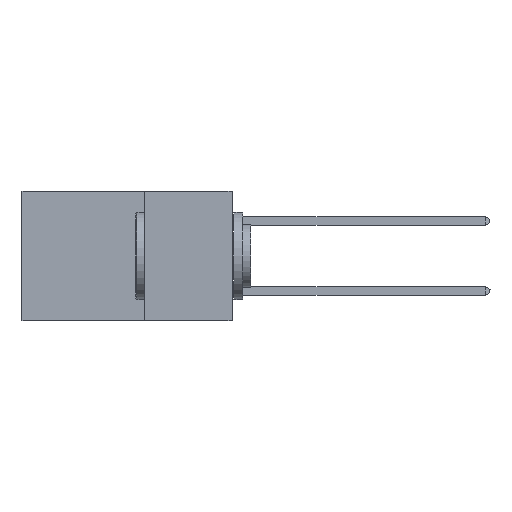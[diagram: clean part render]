
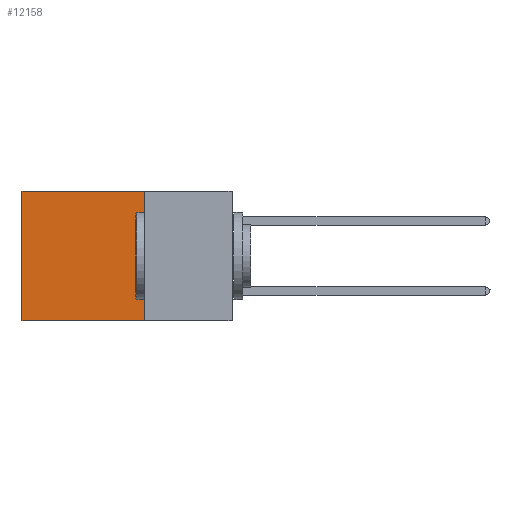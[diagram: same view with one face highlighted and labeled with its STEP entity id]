
A CAD part, left-side view. The second image highlights one B-rep face of the part: STEP entity #12158.
In plain terms, the highlighted planar face has unit normal (-1, 0, 0).
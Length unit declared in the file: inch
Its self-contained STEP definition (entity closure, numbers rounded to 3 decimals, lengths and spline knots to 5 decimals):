
#1408 = CARTESIAN_POINT ( 'NONE',  ( 0.2875, 0.25, 0. ) ) ;
#3060 = VECTOR ( 'NONE', #18854, 39.37008 ) ;
#3437 = ORIENTED_EDGE ( 'NONE', *, *, #14255, .F. ) ;
#5134 = ORIENTED_EDGE ( 'NONE', *, *, #11934, .F. ) ;
#6061 = ORIENTED_EDGE ( 'NONE', *, *, #16814, .T. ) ;
#7436 = FACE_OUTER_BOUND ( 'NONE', #12693, .T. ) ;
#8294 = LINE ( 'NONE', #42386, #42896 ) ;
#11934 = EDGE_CURVE ( 'NONE', #23235, #21359, #41029, .T. ) ;
#12158 = ADVANCED_FACE ( 'NONE', ( #7436 ), #16274, .F. ) ;
#12693 = EDGE_LOOP ( 'NONE', ( #6061, #3437, #5134, #21811 ) ) ;
#12877 = LINE ( 'NONE', #31727, #30169 ) ;
#14255 = EDGE_CURVE ( 'NONE', #21359, #35211, #8294, .T. ) ;
#14597 = LINE ( 'NONE', #27850, #3060 ) ;
#15243 = CARTESIAN_POINT ( 'NONE',  ( 0.2875, 0.6, 0. ) ) ;
#16274 = PLANE ( 'NONE',  #39354 ) ;
#16450 = VECTOR ( 'NONE', #43091, 39.37008 ) ;
#16814 = EDGE_CURVE ( 'NONE', #19203, #35211, #12877, .T. ) ;
#18534 = DIRECTION ( 'NONE',  ( 0., 1., 0. ) ) ;
#18854 = DIRECTION ( 'NONE',  ( 0., 1., 0. ) ) ;
#19203 = VERTEX_POINT ( 'NONE', #15243 ) ;
#19627 = CARTESIAN_POINT ( 'NONE',  ( 0.2875, 0.25, 0. ) ) ;
#19917 = EDGE_CURVE ( 'NONE', #23235, #19203, #14597, .T. ) ;
#21359 = VERTEX_POINT ( 'NONE', #40702 ) ;
#21811 = ORIENTED_EDGE ( 'NONE', *, *, #19917, .T. ) ;
#23235 = VERTEX_POINT ( 'NONE', #33726 ) ;
#26616 = DIRECTION ( 'NONE',  ( 0., 0., -1. ) ) ;
#26856 = CARTESIAN_POINT ( 'NONE',  ( 0.2875, 0.6, -0.37 ) ) ;
#27850 = CARTESIAN_POINT ( 'NONE',  ( 0.2875, 0.25, 0. ) ) ;
#30169 = VECTOR ( 'NONE', #26616, 39.37008 ) ;
#31727 = CARTESIAN_POINT ( 'NONE',  ( 0.2875, 0.6, 0. ) ) ;
#32390 = DIRECTION ( 'NONE',  ( 0., 0., -1. ) ) ;
#33726 = CARTESIAN_POINT ( 'NONE',  ( 0.2875, 0.25, 0. ) ) ;
#35211 = VERTEX_POINT ( 'NONE', #26856 ) ;
#39281 = DIRECTION ( 'NONE',  ( 1., 0., 0. ) ) ;
#39354 = AXIS2_PLACEMENT_3D ( 'NONE', #19627, #39281, #32390 ) ;
#40702 = CARTESIAN_POINT ( 'NONE',  ( 0.2875, 0.25, -0.37 ) ) ;
#41029 = LINE ( 'NONE', #1408, #16450 ) ;
#42386 = CARTESIAN_POINT ( 'NONE',  ( 0.2875, 0.25, -0.37 ) ) ;
#42896 = VECTOR ( 'NONE', #18534, 39.37008 ) ;
#43091 = DIRECTION ( 'NONE',  ( 0., 0., -1. ) ) ;
